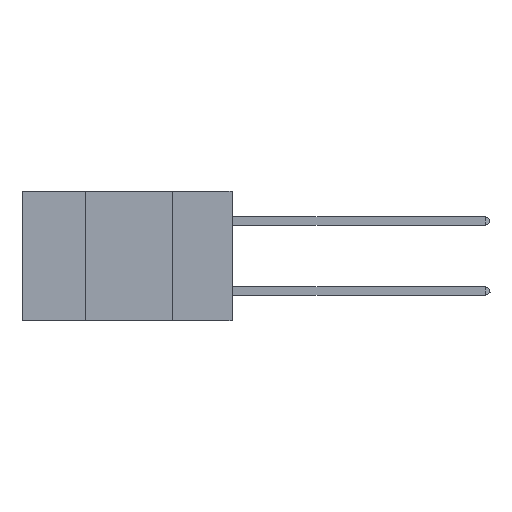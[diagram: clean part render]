
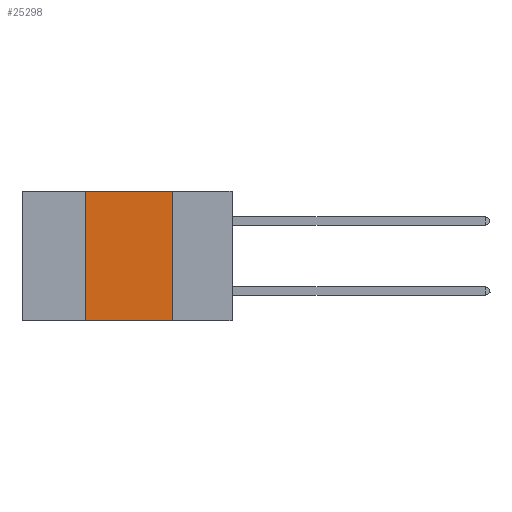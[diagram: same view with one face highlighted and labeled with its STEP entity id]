
A CAD part, left-side view. The second image highlights one B-rep face of the part: STEP entity #25298.
In plain terms, the highlighted planar face has unit normal (-1, 0, 0).
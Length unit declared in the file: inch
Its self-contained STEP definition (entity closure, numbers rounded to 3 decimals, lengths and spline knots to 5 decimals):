
#541 = EDGE_CURVE ( 'NONE', #2200, #20013, #27448, .T. ) ;
#953 = EDGE_CURVE ( 'NONE', #20961, #20013, #15812, .T. ) ;
#1360 = ORIENTED_EDGE ( 'NONE', *, *, #22915, .F. ) ;
#1366 = DIRECTION ( 'NONE',  ( 0., 0., -1. ) ) ;
#1998 = EDGE_LOOP ( 'NONE', ( #15664, #1360, #20239, #10336 ) ) ;
#2200 = VERTEX_POINT ( 'NONE', #12469 ) ;
#4799 = AXIS2_PLACEMENT_3D ( 'NONE', #5711, #10524, #1366 ) ;
#5612 = CARTESIAN_POINT ( 'NONE',  ( 0., 0.17, -0.37 ) ) ;
#5711 = CARTESIAN_POINT ( 'NONE',  ( 0., 0.6, 0. ) ) ;
#6604 = DIRECTION ( 'NONE',  ( 0., -1., 0. ) ) ;
#7192 = VERTEX_POINT ( 'NONE', #25483 ) ;
#8149 = PLANE ( 'NONE',  #4799 ) ;
#8776 = DIRECTION ( 'NONE',  ( 0., 0., -1. ) ) ;
#8929 = VECTOR ( 'NONE', #19005, 39.37008 ) ;
#9313 = CARTESIAN_POINT ( 'NONE',  ( 0., 0.17, 0. ) ) ;
#9448 = VECTOR ( 'NONE', #29172, 39.37008 ) ;
#10336 = ORIENTED_EDGE ( 'NONE', *, *, #541, .T. ) ;
#10524 = DIRECTION ( 'NONE',  ( 1., 0., 0. ) ) ;
#12197 = CARTESIAN_POINT ( 'NONE',  ( 0., 0.6, -0.37 ) ) ;
#12469 = CARTESIAN_POINT ( 'NONE',  ( 0., 0.42, -0.37 ) ) ;
#14933 = LINE ( 'NONE', #21290, #8929 ) ;
#15664 = ORIENTED_EDGE ( 'NONE', *, *, #953, .F. ) ;
#15812 = LINE ( 'NONE', #22196, #22158 ) ;
#19005 = DIRECTION ( 'NONE',  ( 0., 0., 1. ) ) ;
#20013 = VERTEX_POINT ( 'NONE', #5612 ) ;
#20090 = EDGE_CURVE ( 'NONE', #2200, #7192, #14933, .T. ) ;
#20239 = ORIENTED_EDGE ( 'NONE', *, *, #20090, .F. ) ;
#20961 = VERTEX_POINT ( 'NONE', #9313 ) ;
#21290 = CARTESIAN_POINT ( 'NONE',  ( 0., 0.42, 0. ) ) ;
#22158 = VECTOR ( 'NONE', #8776, 39.37008 ) ;
#22196 = CARTESIAN_POINT ( 'NONE',  ( 0., 0.17, 0. ) ) ;
#22915 = EDGE_CURVE ( 'NONE', #7192, #20961, #24597, .T. ) ;
#23725 = FACE_OUTER_BOUND ( 'NONE', #1998, .T. ) ;
#24263 = CARTESIAN_POINT ( 'NONE',  ( 0., 0.6, 0. ) ) ;
#24597 = LINE ( 'NONE', #24263, #26392 ) ;
#25298 = ADVANCED_FACE ( 'NONE', ( #23725 ), #8149, .F. ) ;
#25483 = CARTESIAN_POINT ( 'NONE',  ( 0., 0.42, 0. ) ) ;
#26392 = VECTOR ( 'NONE', #6604, 39.37008 ) ;
#27448 = LINE ( 'NONE', #12197, #9448 ) ;
#29172 = DIRECTION ( 'NONE',  ( 0., -1., 0. ) ) ;
